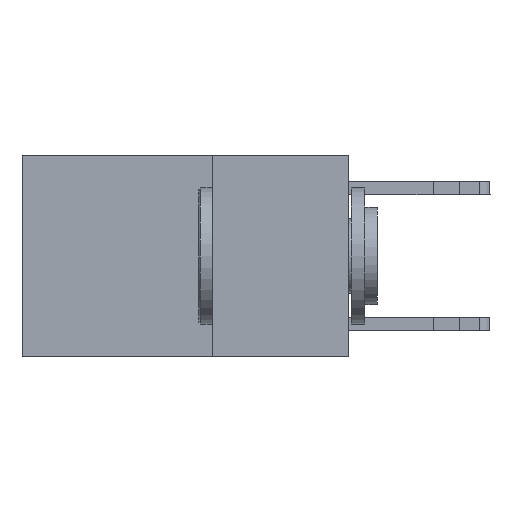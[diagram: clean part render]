
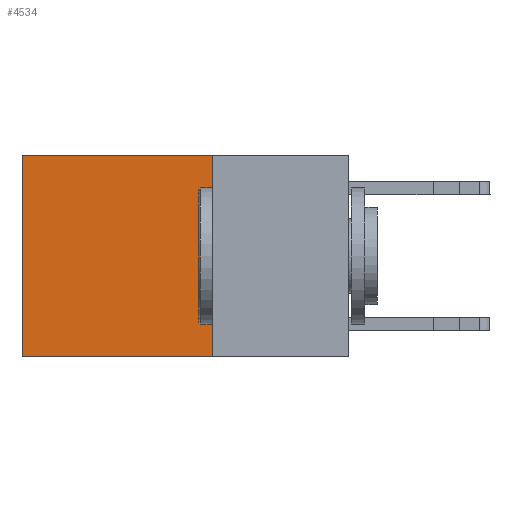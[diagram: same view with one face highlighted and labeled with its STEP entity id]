
A CAD part, left-side view. The second image highlights one B-rep face of the part: STEP entity #4534.
In plain terms, the highlighted planar face has unit normal (-1, 0, 0).
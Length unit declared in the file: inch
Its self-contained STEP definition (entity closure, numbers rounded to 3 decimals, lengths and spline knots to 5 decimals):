
#976 = ORIENTED_EDGE ( 'NONE', *, *, #25373, .T. ) ;
#2299 = ORIENTED_EDGE ( 'NONE', *, *, #4968, .F. ) ;
#2785 = CARTESIAN_POINT ( 'NONE',  ( 0.2625, 0.25, -0.37 ) ) ;
#3642 = DIRECTION ( 'NONE',  ( 1., 0., 0. ) ) ;
#3927 = DIRECTION ( 'NONE',  ( 0., 0., -1. ) ) ;
#4534 = ADVANCED_FACE ( 'NONE', ( #8026 ), #14770, .F. ) ;
#4867 = CARTESIAN_POINT ( 'NONE',  ( 0.2625, 0.6, 0. ) ) ;
#4968 = EDGE_CURVE ( 'NONE', #25617, #16520, #15702, .T. ) ;
#5066 = EDGE_CURVE ( 'NONE', #7873, #26767, #18044, .T. ) ;
#5913 = AXIS2_PLACEMENT_3D ( 'NONE', #16963, #3642, #3927 ) ;
#6314 = CARTESIAN_POINT ( 'NONE',  ( 0.2625, 0.25, 0. ) ) ;
#6906 = DIRECTION ( 'NONE',  ( 0., 0., -1. ) ) ;
#7215 = LINE ( 'NONE', #11614, #12427 ) ;
#7873 = VERTEX_POINT ( 'NONE', #26748 ) ;
#8026 = FACE_OUTER_BOUND ( 'NONE', #14292, .T. ) ;
#10796 = VECTOR ( 'NONE', #6906, 39.37008 ) ;
#11291 = CARTESIAN_POINT ( 'NONE',  ( 0.2625, 0.6, -0.37 ) ) ;
#11384 = VECTOR ( 'NONE', #18932, 39.37008 ) ;
#11614 = CARTESIAN_POINT ( 'NONE',  ( 0.2625, 0.25, 0. ) ) ;
#11755 = DIRECTION ( 'NONE',  ( 0., 1., 0. ) ) ;
#11761 = CARTESIAN_POINT ( 'NONE',  ( 0.2625, 0.25, -0.37 ) ) ;
#12427 = VECTOR ( 'NONE', #11755, 39.37008 ) ;
#12864 = EDGE_CURVE ( 'NONE', #16520, #26767, #16159, .T. ) ;
#13045 = ORIENTED_EDGE ( 'NONE', *, *, #5066, .T. ) ;
#14292 = EDGE_LOOP ( 'NONE', ( #13045, #26628, #2299, #976 ) ) ;
#14770 = PLANE ( 'NONE',  #5913 ) ;
#15135 = DIRECTION ( 'NONE',  ( 0., 0., -1. ) ) ;
#15702 = LINE ( 'NONE', #19666, #21543 ) ;
#16159 = LINE ( 'NONE', #11761, #11384 ) ;
#16520 = VERTEX_POINT ( 'NONE', #2785 ) ;
#16963 = CARTESIAN_POINT ( 'NONE',  ( 0.2625, 0.25, 0. ) ) ;
#18044 = LINE ( 'NONE', #4867, #10796 ) ;
#18932 = DIRECTION ( 'NONE',  ( 0., 1., 0. ) ) ;
#19666 = CARTESIAN_POINT ( 'NONE',  ( 0.2625, 0.25, 0. ) ) ;
#21543 = VECTOR ( 'NONE', #15135, 39.37008 ) ;
#25373 = EDGE_CURVE ( 'NONE', #25617, #7873, #7215, .T. ) ;
#25617 = VERTEX_POINT ( 'NONE', #6314 ) ;
#26628 = ORIENTED_EDGE ( 'NONE', *, *, #12864, .F. ) ;
#26748 = CARTESIAN_POINT ( 'NONE',  ( 0.2625, 0.6, 0. ) ) ;
#26767 = VERTEX_POINT ( 'NONE', #11291 ) ;
